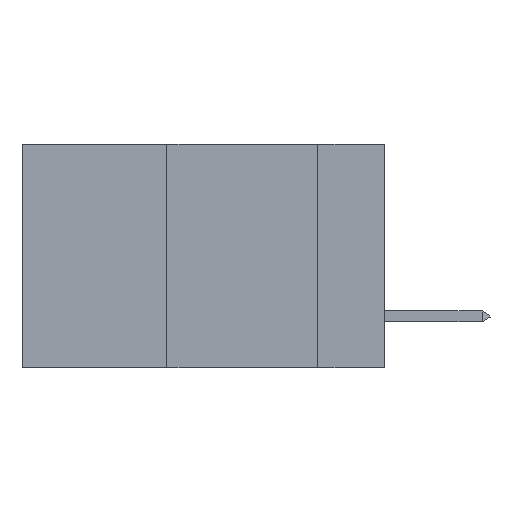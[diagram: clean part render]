
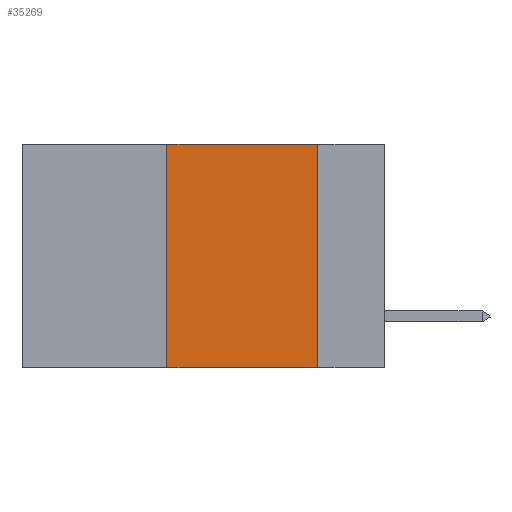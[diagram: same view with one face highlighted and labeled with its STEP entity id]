
A CAD part, left-side view. The second image highlights one B-rep face of the part: STEP entity #35269.
In plain terms, the highlighted planar face has unit normal (-1, 0, 0).
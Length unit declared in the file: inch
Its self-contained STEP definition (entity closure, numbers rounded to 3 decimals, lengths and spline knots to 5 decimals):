
#790 = LINE ( 'NONE', #28263, #26316 ) ;
#1756 = EDGE_CURVE ( 'NONE', #12164, #16902, #26691, .T. ) ;
#1945 = CARTESIAN_POINT ( 'NONE',  ( 0., 0.36, -0.37 ) ) ;
#2318 = ORIENTED_EDGE ( 'NONE', *, *, #10608, .F. ) ;
#2442 = EDGE_LOOP ( 'NONE', ( #36542, #29568, #2318, #11433 ) ) ;
#2964 = DIRECTION ( 'NONE',  ( 0., 0., -1. ) ) ;
#3122 = VECTOR ( 'NONE', #7957, 39.37008 ) ;
#7957 = DIRECTION ( 'NONE',  ( 0., -1., 0. ) ) ;
#8718 = LINE ( 'NONE', #15388, #39502 ) ;
#9139 = CARTESIAN_POINT ( 'NONE',  ( 0., 0.36, 0. ) ) ;
#10608 = EDGE_CURVE ( 'NONE', #13990, #36881, #790, .T. ) ;
#11433 = ORIENTED_EDGE ( 'NONE', *, *, #30018, .T. ) ;
#12164 = VERTEX_POINT ( 'NONE', #15175 ) ;
#13990 = VERTEX_POINT ( 'NONE', #1945 ) ;
#15175 = CARTESIAN_POINT ( 'NONE',  ( 0., 0.11, 0. ) ) ;
#15388 = CARTESIAN_POINT ( 'NONE',  ( 0., 0.6, 0. ) ) ;
#16902 = VERTEX_POINT ( 'NONE', #37424 ) ;
#17584 = CARTESIAN_POINT ( 'NONE',  ( 0., 0.6, 0. ) ) ;
#20786 = DIRECTION ( 'NONE',  ( 1., 0., 0. ) ) ;
#25691 = DIRECTION ( 'NONE',  ( 0., 0., 1. ) ) ;
#26316 = VECTOR ( 'NONE', #25691, 39.37008 ) ;
#26691 = LINE ( 'NONE', #26851, #35376 ) ;
#26851 = CARTESIAN_POINT ( 'NONE',  ( 0., 0.11, 0. ) ) ;
#28020 = FACE_OUTER_BOUND ( 'NONE', #2442, .T. ) ;
#28263 = CARTESIAN_POINT ( 'NONE',  ( 0., 0.36, 0. ) ) ;
#28557 = LINE ( 'NONE', #29269, #3122 ) ;
#29269 = CARTESIAN_POINT ( 'NONE',  ( 0., 0.6, -0.37 ) ) ;
#29568 = ORIENTED_EDGE ( 'NONE', *, *, #32806, .F. ) ;
#30018 = EDGE_CURVE ( 'NONE', #13990, #16902, #28557, .T. ) ;
#31579 = AXIS2_PLACEMENT_3D ( 'NONE', #17584, #20786, #35808 ) ;
#32806 = EDGE_CURVE ( 'NONE', #36881, #12164, #8718, .T. ) ;
#35269 = ADVANCED_FACE ( 'NONE', ( #28020 ), #35673, .F. ) ;
#35376 = VECTOR ( 'NONE', #2964, 39.37008 ) ;
#35673 = PLANE ( 'NONE',  #31579 ) ;
#35808 = DIRECTION ( 'NONE',  ( 0., 0., -1. ) ) ;
#36479 = DIRECTION ( 'NONE',  ( 0., -1., 0. ) ) ;
#36542 = ORIENTED_EDGE ( 'NONE', *, *, #1756, .F. ) ;
#36881 = VERTEX_POINT ( 'NONE', #9139 ) ;
#37424 = CARTESIAN_POINT ( 'NONE',  ( 0., 0.11, -0.37 ) ) ;
#39502 = VECTOR ( 'NONE', #36479, 39.37008 ) ;
